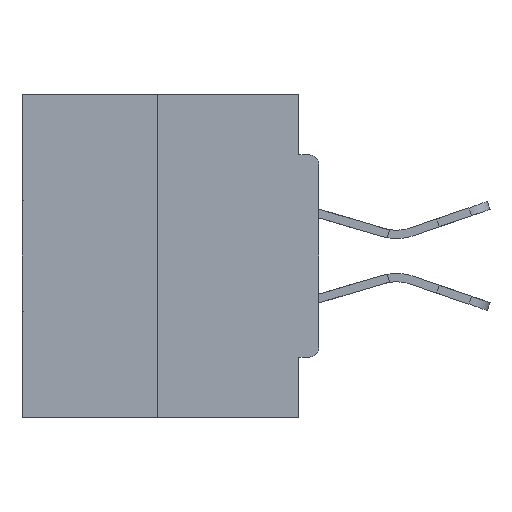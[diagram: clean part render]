
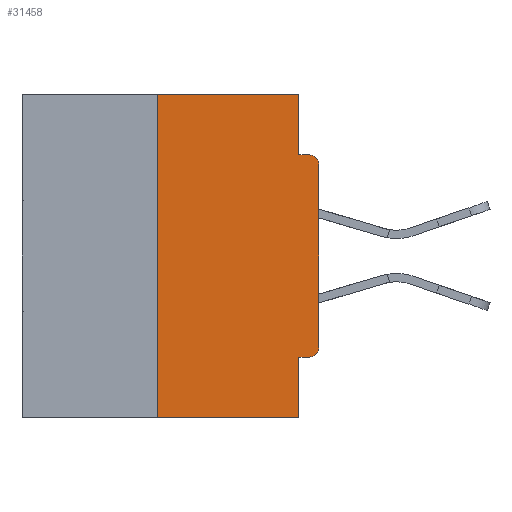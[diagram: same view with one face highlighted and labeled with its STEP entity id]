
A CAD part, left-side view. The second image highlights one B-rep face of the part: STEP entity #31458.
In plain terms, the highlighted planar face has unit normal (-1, 0, 0).
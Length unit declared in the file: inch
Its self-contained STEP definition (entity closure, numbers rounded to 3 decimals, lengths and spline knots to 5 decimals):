
#363 = DIRECTION ( 'NONE',  ( -1., 0., 0. ) ) ;
#693 = LINE ( 'NONE', #21149, #13427 ) ;
#924 = DIRECTION ( 'NONE',  ( 0., 0., -1. ) ) ;
#988 = EDGE_CURVE ( 'NONE', #7704, #7282, #8747, .T. ) ;
#1846 = CIRCLE ( 'NONE', #28822, 0.015 ) ;
#1884 = CARTESIAN_POINT ( 'NONE',  ( 0., 0.031, 0. ) ) ;
#2130 = EDGE_CURVE ( 'NONE', #10889, #34721, #16081, .T. ) ;
#2856 = CARTESIAN_POINT ( 'NONE',  ( 0., 0., -0.0935 ) ) ;
#2978 = CARTESIAN_POINT ( 'NONE',  ( 0., 0.031, 0. ) ) ;
#3025 = DIRECTION ( 'NONE',  ( 0., 0., 1. ) ) ;
#3755 = VERTEX_POINT ( 'NONE', #1884 ) ;
#4128 = CARTESIAN_POINT ( 'NONE',  ( 0., 0., -0.4065 ) ) ;
#4293 = ORIENTED_EDGE ( 'NONE', *, *, #35214, .T. ) ;
#4359 = CARTESIAN_POINT ( 'NONE',  ( 0., 0., -0.1085 ) ) ;
#4876 = VECTOR ( 'NONE', #32193, 39.37008 ) ;
#6216 = DIRECTION ( 'NONE',  ( 0., 0., 1. ) ) ;
#6636 = CARTESIAN_POINT ( 'NONE',  ( 0., 0.46, 0. ) ) ;
#6655 = LINE ( 'NONE', #30416, #32243 ) ;
#6755 = AXIS2_PLACEMENT_3D ( 'NONE', #6636, #9188, #9753 ) ;
#6816 = CARTESIAN_POINT ( 'NONE',  ( 0., 0.031, -0.5 ) ) ;
#7282 = VERTEX_POINT ( 'NONE', #8556 ) ;
#7704 = VERTEX_POINT ( 'NONE', #32495 ) ;
#7855 = CARTESIAN_POINT ( 'NONE',  ( 0., 0.031, -0.5 ) ) ;
#8423 = ORIENTED_EDGE ( 'NONE', *, *, #36580, .F. ) ;
#8556 = CARTESIAN_POINT ( 'NONE',  ( 0., 0.015, -0.0935 ) ) ;
#8747 = LINE ( 'NONE', #2856, #9212 ) ;
#9188 = DIRECTION ( 'NONE',  ( 1., 0., 0. ) ) ;
#9212 = VECTOR ( 'NONE', #29759, 39.37008 ) ;
#9269 = EDGE_CURVE ( 'NONE', #34721, #20852, #21750, .T. ) ;
#9753 = DIRECTION ( 'NONE',  ( 0., 0., -1. ) ) ;
#10154 = DIRECTION ( 'NONE',  ( 0., -1., 0. ) ) ;
#10695 = CARTESIAN_POINT ( 'NONE',  ( 0., 0.015, -0.1085 ) ) ;
#10748 = CARTESIAN_POINT ( 'NONE',  ( 0., 0.031, -0.4065 ) ) ;
#10889 = VERTEX_POINT ( 'NONE', #38109 ) ;
#11148 = CARTESIAN_POINT ( 'NONE',  ( 0., 0.46, 0. ) ) ;
#11813 = AXIS2_PLACEMENT_3D ( 'NONE', #21383, #363, #924 ) ;
#11845 = CARTESIAN_POINT ( 'NONE',  ( 0., 0.25, 0. ) ) ;
#12765 = LINE ( 'NONE', #2978, #25433 ) ;
#13088 = DIRECTION ( 'NONE',  ( 0., 0., -1. ) ) ;
#13427 = VECTOR ( 'NONE', #6216, 39.37008 ) ;
#13651 = DIRECTION ( 'NONE',  ( -1., 0., 0. ) ) ;
#15269 = PLANE ( 'NONE',  #6755 ) ;
#15753 = CARTESIAN_POINT ( 'NONE',  ( 0., 0.25, 0. ) ) ;
#16081 = LINE ( 'NONE', #4128, #19302 ) ;
#16257 = ORIENTED_EDGE ( 'NONE', *, *, #31253, .F. ) ;
#18932 = EDGE_CURVE ( 'NONE', #23040, #32471, #26600, .T. ) ;
#19302 = VECTOR ( 'NONE', #28261, 39.37008 ) ;
#19341 = DIRECTION ( 'NONE',  ( 0., 0., -1. ) ) ;
#19884 = ORIENTED_EDGE ( 'NONE', *, *, #32777, .T. ) ;
#20398 = LINE ( 'NONE', #11148, #4876 ) ;
#20623 = VERTEX_POINT ( 'NONE', #35590 ) ;
#20852 = VERTEX_POINT ( 'NONE', #7855 ) ;
#21056 = DIRECTION ( 'NONE',  ( 0., 0., -1. ) ) ;
#21149 = CARTESIAN_POINT ( 'NONE',  ( 0., 0., 0. ) ) ;
#21383 = CARTESIAN_POINT ( 'NONE',  ( 0., 0.015, -0.3915 ) ) ;
#21750 = LINE ( 'NONE', #6816, #23929 ) ;
#22208 = ORIENTED_EDGE ( 'NONE', *, *, #18932, .F. ) ;
#22452 = ORIENTED_EDGE ( 'NONE', *, *, #2130, .F. ) ;
#22720 = VECTOR ( 'NONE', #3025, 39.37008 ) ;
#23040 = VERTEX_POINT ( 'NONE', #32327 ) ;
#23929 = VECTOR ( 'NONE', #13088, 39.37008 ) ;
#23988 = ORIENTED_EDGE ( 'NONE', *, *, #33301, .T. ) ;
#25433 = VECTOR ( 'NONE', #21056, 39.37008 ) ;
#26600 = LINE ( 'NONE', #11845, #22720 ) ;
#26750 = VERTEX_POINT ( 'NONE', #4359 ) ;
#28261 = DIRECTION ( 'NONE',  ( 0., 1., 0. ) ) ;
#28768 = CIRCLE ( 'NONE', #11813, 0.015 ) ;
#28822 = AXIS2_PLACEMENT_3D ( 'NONE', #10695, #13651, #19341 ) ;
#29759 = DIRECTION ( 'NONE',  ( 0., -1., 0. ) ) ;
#30416 = CARTESIAN_POINT ( 'NONE',  ( 0., 0.46, -0.5 ) ) ;
#30485 = EDGE_LOOP ( 'NONE', ( #16257, #22208, #33500, #30659, #22452, #19884, #4293, #23988, #34761, #8423 ) ) ;
#30659 = ORIENTED_EDGE ( 'NONE', *, *, #9269, .F. ) ;
#31253 = EDGE_CURVE ( 'NONE', #32471, #3755, #20398, .T. ) ;
#31458 = ADVANCED_FACE ( 'NONE', ( #36313 ), #15269, .F. ) ;
#32193 = DIRECTION ( 'NONE',  ( 0., -1., 0. ) ) ;
#32243 = VECTOR ( 'NONE', #10154, 39.37008 ) ;
#32327 = CARTESIAN_POINT ( 'NONE',  ( 0., 0.25, -0.5 ) ) ;
#32471 = VERTEX_POINT ( 'NONE', #15753 ) ;
#32495 = CARTESIAN_POINT ( 'NONE',  ( 0., 0.031, -0.0935 ) ) ;
#32777 = EDGE_CURVE ( 'NONE', #10889, #20623, #28768, .T. ) ;
#33301 = EDGE_CURVE ( 'NONE', #26750, #7282, #1846, .T. ) ;
#33500 = ORIENTED_EDGE ( 'NONE', *, *, #34643, .T. ) ;
#34643 = EDGE_CURVE ( 'NONE', #23040, #20852, #6655, .T. ) ;
#34721 = VERTEX_POINT ( 'NONE', #10748 ) ;
#34761 = ORIENTED_EDGE ( 'NONE', *, *, #988, .F. ) ;
#35214 = EDGE_CURVE ( 'NONE', #20623, #26750, #693, .T. ) ;
#35590 = CARTESIAN_POINT ( 'NONE',  ( 0., 0., -0.3915 ) ) ;
#36313 = FACE_OUTER_BOUND ( 'NONE', #30485, .T. ) ;
#36580 = EDGE_CURVE ( 'NONE', #3755, #7704, #12765, .T. ) ;
#38109 = CARTESIAN_POINT ( 'NONE',  ( 0., 0.015, -0.4065 ) ) ;
